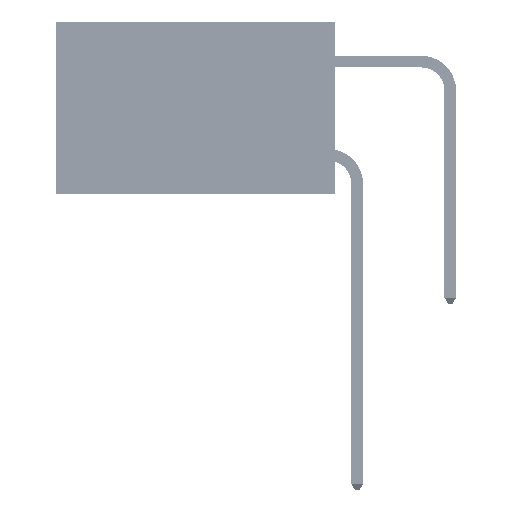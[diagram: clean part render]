
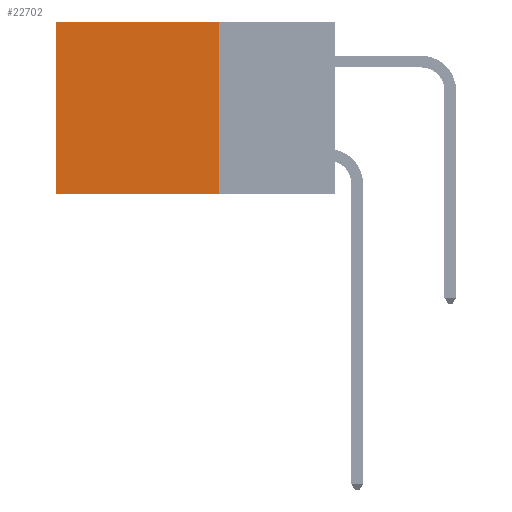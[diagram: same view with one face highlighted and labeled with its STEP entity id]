
A CAD part, left-side view. The second image highlights one B-rep face of the part: STEP entity #22702.
In plain terms, the highlighted planar face has unit normal (-1, 0, 0).
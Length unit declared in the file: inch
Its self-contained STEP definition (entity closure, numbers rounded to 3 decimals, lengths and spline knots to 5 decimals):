
#1284 = CARTESIAN_POINT ( 'NONE',  ( 0.2875, 0.25, -0.37 ) ) ;
#2070 = CARTESIAN_POINT ( 'NONE',  ( 0.2875, 0.6, -0.37 ) ) ;
#2737 = FACE_OUTER_BOUND ( 'NONE', #18645, .T. ) ;
#3721 = EDGE_CURVE ( 'NONE', #16602, #43795, #15919, .T. ) ;
#4005 = VECTOR ( 'NONE', #25245, 39.37008 ) ;
#5701 = CARTESIAN_POINT ( 'NONE',  ( 0.2875, 0.6, 0. ) ) ;
#8817 = LINE ( 'NONE', #15650, #42173 ) ;
#9618 = CARTESIAN_POINT ( 'NONE',  ( 0.2875, 0.25, -0.37 ) ) ;
#10271 = DIRECTION ( 'NONE',  ( 1., 0., 0. ) ) ;
#10411 = VERTEX_POINT ( 'NONE', #5701 ) ;
#15650 = CARTESIAN_POINT ( 'NONE',  ( 0.2875, 0.25, 0. ) ) ;
#15919 = LINE ( 'NONE', #1284, #18196 ) ;
#16602 = VERTEX_POINT ( 'NONE', #9618 ) ;
#17603 = PLANE ( 'NONE',  #34967 ) ;
#18196 = VECTOR ( 'NONE', #30973, 39.37008 ) ;
#18645 = EDGE_LOOP ( 'NONE', ( #45019, #22331, #43318, #27122 ) ) ;
#21062 = LINE ( 'NONE', #21308, #36002 ) ;
#21308 = CARTESIAN_POINT ( 'NONE',  ( 0.2875, 0.6, 0. ) ) ;
#22331 = ORIENTED_EDGE ( 'NONE', *, *, #3721, .F. ) ;
#22702 = ADVANCED_FACE ( 'NONE', ( #2737 ), #17603, .F. ) ;
#25245 = DIRECTION ( 'NONE',  ( 0., 0., -1. ) ) ;
#25293 = EDGE_CURVE ( 'NONE', #35051, #16602, #32298, .T. ) ;
#25436 = DIRECTION ( 'NONE',  ( 0., 0., -1. ) ) ;
#27122 = ORIENTED_EDGE ( 'NONE', *, *, #30786, .T. ) ;
#28242 = CARTESIAN_POINT ( 'NONE',  ( 0.2875, 0.25, 0. ) ) ;
#30473 = DIRECTION ( 'NONE',  ( 0., 1., 0. ) ) ;
#30786 = EDGE_CURVE ( 'NONE', #35051, #10411, #8817, .T. ) ;
#30973 = DIRECTION ( 'NONE',  ( 0., 1., 0. ) ) ;
#32298 = LINE ( 'NONE', #43979, #4005 ) ;
#32423 = CARTESIAN_POINT ( 'NONE',  ( 0.2875, 0.25, 0. ) ) ;
#34967 = AXIS2_PLACEMENT_3D ( 'NONE', #32423, #10271, #41402 ) ;
#35051 = VERTEX_POINT ( 'NONE', #28242 ) ;
#36002 = VECTOR ( 'NONE', #25436, 39.37008 ) ;
#41402 = DIRECTION ( 'NONE',  ( 0., 0., -1. ) ) ;
#42173 = VECTOR ( 'NONE', #30473, 39.37008 ) ;
#43318 = ORIENTED_EDGE ( 'NONE', *, *, #25293, .F. ) ;
#43795 = VERTEX_POINT ( 'NONE', #2070 ) ;
#43979 = CARTESIAN_POINT ( 'NONE',  ( 0.2875, 0.25, 0. ) ) ;
#43985 = EDGE_CURVE ( 'NONE', #10411, #43795, #21062, .T. ) ;
#45019 = ORIENTED_EDGE ( 'NONE', *, *, #43985, .T. ) ;
